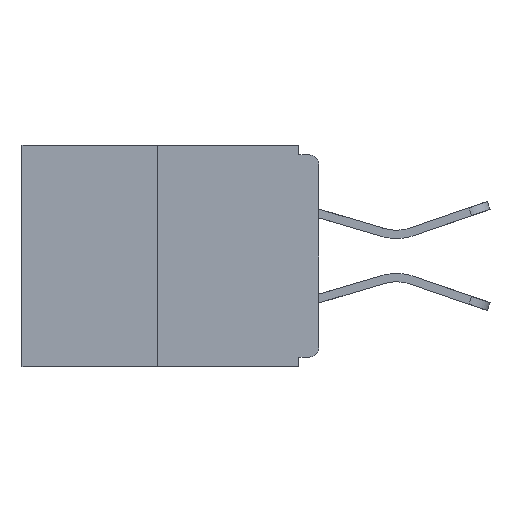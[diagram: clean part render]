
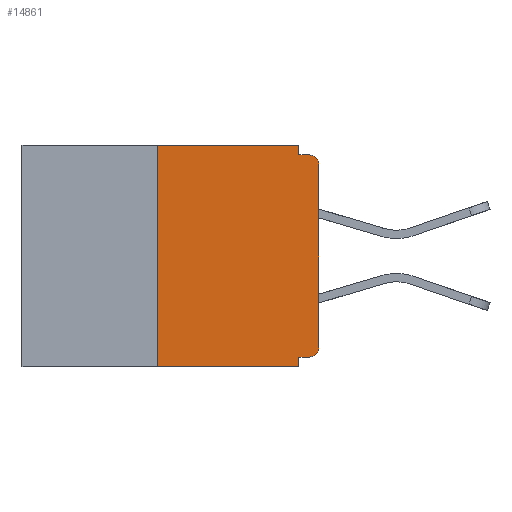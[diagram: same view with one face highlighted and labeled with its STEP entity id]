
A CAD part, left-side view. The second image highlights one B-rep face of the part: STEP entity #14861.
In plain terms, the highlighted planar face has unit normal (-1, 0, 0).
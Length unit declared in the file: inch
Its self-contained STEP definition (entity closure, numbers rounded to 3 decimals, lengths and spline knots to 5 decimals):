
#351 = CARTESIAN_POINT ( 'NONE',  ( 0., 0.015, -0.03 ) ) ;
#730 = DIRECTION ( 'NONE',  ( 0., 0., 1. ) ) ;
#921 = CARTESIAN_POINT ( 'NONE',  ( 0., 0.031, -0.343 ) ) ;
#1320 = LINE ( 'NONE', #3747, #12253 ) ;
#1659 = AXIS2_PLACEMENT_3D ( 'NONE', #30159, #5487, #10398 ) ;
#1746 = CARTESIAN_POINT ( 'NONE',  ( 0., 0.031, -0.343 ) ) ;
#1815 = LINE ( 'NONE', #1746, #2980 ) ;
#1993 = VERTEX_POINT ( 'NONE', #23694 ) ;
#2319 = EDGE_CURVE ( 'NONE', #4304, #30179, #1320, .T. ) ;
#2646 = CARTESIAN_POINT ( 'NONE',  ( 0., 0.015, -0.328 ) ) ;
#2980 = VECTOR ( 'NONE', #12112, 39.37008 ) ;
#2981 = PLANE ( 'NONE',  #1659 ) ;
#3747 = CARTESIAN_POINT ( 'NONE',  ( 0., 0.46, -0.343 ) ) ;
#3791 = VERTEX_POINT ( 'NONE', #2646 ) ;
#4004 = CARTESIAN_POINT ( 'NONE',  ( 0., 0.25, 0. ) ) ;
#4295 = AXIS2_PLACEMENT_3D ( 'NONE', #351, #27664, #24912 ) ;
#4304 = VERTEX_POINT ( 'NONE', #16786 ) ;
#4349 = CARTESIAN_POINT ( 'NONE',  ( 0., 0.46, 0. ) ) ;
#5487 = DIRECTION ( 'NONE',  ( 1., 0., 0. ) ) ;
#6466 = EDGE_CURVE ( 'NONE', #1993, #30179, #1815, .T. ) ;
#7194 = CARTESIAN_POINT ( 'NONE',  ( 0., 0.25, 0. ) ) ;
#7657 = VECTOR ( 'NONE', #27707, 39.37008 ) ;
#8511 = DIRECTION ( 'NONE',  ( 0., -1., 0. ) ) ;
#8528 = DIRECTION ( 'NONE',  ( 0., 0., -1. ) ) ;
#8780 = VERTEX_POINT ( 'NONE', #27772 ) ;
#9187 = EDGE_CURVE ( 'NONE', #12396, #32004, #28752, .T. ) ;
#9329 = ORIENTED_EDGE ( 'NONE', *, *, #18911, .F. ) ;
#10226 = AXIS2_PLACEMENT_3D ( 'NONE', #18431, #11062, #8528 ) ;
#10398 = DIRECTION ( 'NONE',  ( 0., 0., -1. ) ) ;
#10969 = CARTESIAN_POINT ( 'NONE',  ( 0., 0.031, 0. ) ) ;
#11062 = DIRECTION ( 'NONE',  ( -1., 0., 0. ) ) ;
#11064 = EDGE_CURVE ( 'NONE', #30329, #15436, #16688, .T. ) ;
#11245 = VECTOR ( 'NONE', #730, 39.37008 ) ;
#11337 = EDGE_CURVE ( 'NONE', #27819, #30329, #27108, .T. ) ;
#12112 = DIRECTION ( 'NONE',  ( 0., 0., -1. ) ) ;
#12253 = VECTOR ( 'NONE', #8511, 39.37008 ) ;
#12396 = VERTEX_POINT ( 'NONE', #4004 ) ;
#12813 = LINE ( 'NONE', #23521, #19039 ) ;
#13545 = LINE ( 'NONE', #27506, #7657 ) ;
#14628 = EDGE_CURVE ( 'NONE', #8780, #15436, #13545, .T. ) ;
#14739 = LINE ( 'NONE', #10969, #25557 ) ;
#14861 = ADVANCED_FACE ( 'NONE', ( #29712 ), #2981, .F. ) ;
#15201 = VECTOR ( 'NONE', #29442, 39.37008 ) ;
#15436 = VERTEX_POINT ( 'NONE', #22455 ) ;
#15503 = ORIENTED_EDGE ( 'NONE', *, *, #11064, .T. ) ;
#15567 = VECTOR ( 'NONE', #24274, 39.37008 ) ;
#16384 = CARTESIAN_POINT ( 'NONE',  ( 0., 0., -0.03 ) ) ;
#16688 = CIRCLE ( 'NONE', #4295, 0.015 ) ;
#16786 = CARTESIAN_POINT ( 'NONE',  ( 0., 0.25, -0.343 ) ) ;
#16897 = ORIENTED_EDGE ( 'NONE', *, *, #19744, .F. ) ;
#17099 = ORIENTED_EDGE ( 'NONE', *, *, #14628, .F. ) ;
#17284 = ORIENTED_EDGE ( 'NONE', *, *, #6466, .F. ) ;
#18431 = CARTESIAN_POINT ( 'NONE',  ( 0., 0.015, -0.313 ) ) ;
#18911 = EDGE_CURVE ( 'NONE', #4304, #12396, #22152, .T. ) ;
#19039 = VECTOR ( 'NONE', #20667, 39.37008 ) ;
#19744 = EDGE_CURVE ( 'NONE', #3791, #1993, #12813, .T. ) ;
#20139 = EDGE_CURVE ( 'NONE', #32004, #8780, #14739, .T. ) ;
#20667 = DIRECTION ( 'NONE',  ( 0., 1., 0. ) ) ;
#22152 = LINE ( 'NONE', #7194, #15567 ) ;
#22455 = CARTESIAN_POINT ( 'NONE',  ( 0., 0.015, -0.015 ) ) ;
#23521 = CARTESIAN_POINT ( 'NONE',  ( 0., 0., -0.328 ) ) ;
#23601 = EDGE_LOOP ( 'NONE', ( #26921, #9329, #30229, #17284, #16897, #24457, #31109, #15503, #17099, #27520 ) ) ;
#23694 = CARTESIAN_POINT ( 'NONE',  ( 0., 0.031, -0.328 ) ) ;
#24033 = CARTESIAN_POINT ( 'NONE',  ( 0., 0., -0.313 ) ) ;
#24044 = CARTESIAN_POINT ( 'NONE',  ( 0., 0., 0. ) ) ;
#24274 = DIRECTION ( 'NONE',  ( 0., 0., 1. ) ) ;
#24457 = ORIENTED_EDGE ( 'NONE', *, *, #25763, .T. ) ;
#24912 = DIRECTION ( 'NONE',  ( 0., 0., -1. ) ) ;
#24966 = CIRCLE ( 'NONE', #10226, 0.015 ) ;
#25557 = VECTOR ( 'NONE', #28251, 39.37008 ) ;
#25763 = EDGE_CURVE ( 'NONE', #3791, #27819, #24966, .T. ) ;
#26921 = ORIENTED_EDGE ( 'NONE', *, *, #9187, .F. ) ;
#27108 = LINE ( 'NONE', #24044, #11245 ) ;
#27506 = CARTESIAN_POINT ( 'NONE',  ( 0., 0., -0.015 ) ) ;
#27520 = ORIENTED_EDGE ( 'NONE', *, *, #20139, .F. ) ;
#27664 = DIRECTION ( 'NONE',  ( -1., 0., 0. ) ) ;
#27707 = DIRECTION ( 'NONE',  ( 0., -1., 0. ) ) ;
#27772 = CARTESIAN_POINT ( 'NONE',  ( 0., 0.031, -0.015 ) ) ;
#27819 = VERTEX_POINT ( 'NONE', #24033 ) ;
#28251 = DIRECTION ( 'NONE',  ( 0., 0., -1. ) ) ;
#28752 = LINE ( 'NONE', #4349, #15201 ) ;
#29442 = DIRECTION ( 'NONE',  ( 0., -1., 0. ) ) ;
#29712 = FACE_OUTER_BOUND ( 'NONE', #23601, .T. ) ;
#29767 = CARTESIAN_POINT ( 'NONE',  ( 0., 0.031, 0. ) ) ;
#30159 = CARTESIAN_POINT ( 'NONE',  ( 0., 0.46, 0. ) ) ;
#30179 = VERTEX_POINT ( 'NONE', #921 ) ;
#30229 = ORIENTED_EDGE ( 'NONE', *, *, #2319, .T. ) ;
#30329 = VERTEX_POINT ( 'NONE', #16384 ) ;
#31109 = ORIENTED_EDGE ( 'NONE', *, *, #11337, .T. ) ;
#32004 = VERTEX_POINT ( 'NONE', #29767 ) ;
